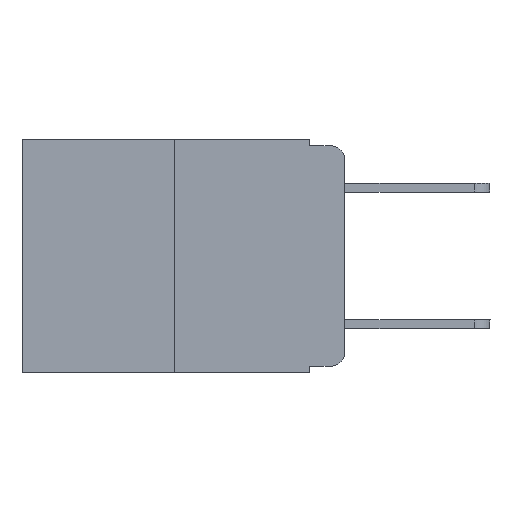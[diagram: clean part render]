
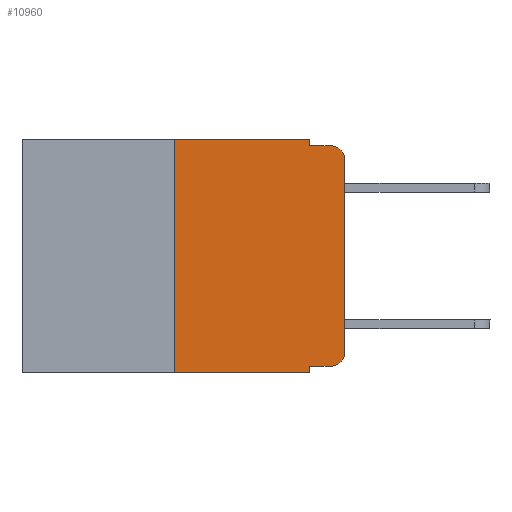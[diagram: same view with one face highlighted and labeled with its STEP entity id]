
A CAD part, left-side view. The second image highlights one B-rep face of the part: STEP entity #10960.
In plain terms, the highlighted planar face has unit normal (-1, 0, 0).
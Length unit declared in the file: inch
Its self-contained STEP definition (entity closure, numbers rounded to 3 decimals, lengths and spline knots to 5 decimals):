
#119 = LINE ( 'NONE', #8763, #12037 ) ;
#389 = VECTOR ( 'NONE', #10071, 39.37008 ) ;
#636 = CARTESIAN_POINT ( 'NONE',  ( 0., 0., -0.03 ) ) ;
#895 = DIRECTION ( 'NONE',  ( 0., 0., 1. ) ) ;
#909 = DIRECTION ( 'NONE',  ( 1., 0., 0. ) ) ;
#919 = VERTEX_POINT ( 'NONE', #2746 ) ;
#997 = CARTESIAN_POINT ( 'NONE',  ( 0., 0.473, 0. ) ) ;
#1603 = CARTESIAN_POINT ( 'NONE',  ( 0., 0.051, -0.333 ) ) ;
#1807 = LINE ( 'NONE', #5413, #7610 ) ;
#1819 = ORIENTED_EDGE ( 'NONE', *, *, #3888, .T. ) ;
#2052 = LINE ( 'NONE', #9664, #5678 ) ;
#2224 = DIRECTION ( 'NONE',  ( 0., -1., 0. ) ) ;
#2333 = CARTESIAN_POINT ( 'NONE',  ( 0., 0.051, -0.01 ) ) ;
#2435 = VERTEX_POINT ( 'NONE', #2333 ) ;
#2512 = VERTEX_POINT ( 'NONE', #636 ) ;
#2543 = DIRECTION ( 'NONE',  ( 0., 0., -1. ) ) ;
#2651 = AXIS2_PLACEMENT_3D ( 'NONE', #4947, #2930, #3047 ) ;
#2669 = CARTESIAN_POINT ( 'NONE',  ( 0., 0.02, -0.333 ) ) ;
#2746 = CARTESIAN_POINT ( 'NONE',  ( 0., 0.02, -0.01 ) ) ;
#2767 = ORIENTED_EDGE ( 'NONE', *, *, #9266, .T. ) ;
#2859 = LINE ( 'NONE', #11042, #389 ) ;
#2873 = LINE ( 'NONE', #8002, #8405 ) ;
#2891 = DIRECTION ( 'NONE',  ( 0., 0., -1. ) ) ;
#2930 = DIRECTION ( 'NONE',  ( -1., 0., 0. ) ) ;
#3047 = DIRECTION ( 'NONE',  ( 0., 0., -1. ) ) ;
#3244 = VECTOR ( 'NONE', #895, 39.37008 ) ;
#3314 = VERTEX_POINT ( 'NONE', #1603 ) ;
#3888 = EDGE_CURVE ( 'NONE', #2512, #919, #4780, .T. ) ;
#3894 = VECTOR ( 'NONE', #5170, 39.37008 ) ;
#4258 = VERTEX_POINT ( 'NONE', #10724 ) ;
#4780 = CIRCLE ( 'NONE', #5153, 0.02 ) ;
#4947 = CARTESIAN_POINT ( 'NONE',  ( 0., 0.02, -0.313 ) ) ;
#5011 = EDGE_CURVE ( 'NONE', #7599, #4258, #5187, .T. ) ;
#5047 = VERTEX_POINT ( 'NONE', #8077 ) ;
#5153 = AXIS2_PLACEMENT_3D ( 'NONE', #9343, #11237, #2891 ) ;
#5170 = DIRECTION ( 'NONE',  ( 0., 0., 1. ) ) ;
#5187 = LINE ( 'NONE', #8917, #3894 ) ;
#5374 = AXIS2_PLACEMENT_3D ( 'NONE', #997, #909, #7521 ) ;
#5413 = CARTESIAN_POINT ( 'NONE',  ( 0., 0.051, -0.01 ) ) ;
#5415 = ORIENTED_EDGE ( 'NONE', *, *, #7147, .F. ) ;
#5508 = ORIENTED_EDGE ( 'NONE', *, *, #11428, .T. ) ;
#5583 = CARTESIAN_POINT ( 'NONE',  ( 0., 0.25, -0.343 ) ) ;
#5678 = VECTOR ( 'NONE', #9786, 39.37008 ) ;
#5711 = CARTESIAN_POINT ( 'NONE',  ( 0., 0.473, 0. ) ) ;
#6020 = EDGE_CURVE ( 'NONE', #5047, #2435, #2859, .T. ) ;
#6319 = ORIENTED_EDGE ( 'NONE', *, *, #6020, .F. ) ;
#6536 = PLANE ( 'NONE',  #5374 ) ;
#6649 = DIRECTION ( 'NONE',  ( 0., -1., 0. ) ) ;
#6833 = CARTESIAN_POINT ( 'NONE',  ( 0., 0., -0.313 ) ) ;
#7147 = EDGE_CURVE ( 'NONE', #4258, #5047, #11129, .T. ) ;
#7521 = DIRECTION ( 'NONE',  ( 0., 0., -1. ) ) ;
#7543 = EDGE_CURVE ( 'NONE', #2435, #919, #1807, .T. ) ;
#7599 = VERTEX_POINT ( 'NONE', #5583 ) ;
#7610 = VECTOR ( 'NONE', #11765, 39.37008 ) ;
#7619 = EDGE_CURVE ( 'NONE', #10535, #2512, #9797, .T. ) ;
#7634 = ORIENTED_EDGE ( 'NONE', *, *, #7543, .F. ) ;
#8002 = CARTESIAN_POINT ( 'NONE',  ( 0., 0.051, 0. ) ) ;
#8077 = CARTESIAN_POINT ( 'NONE',  ( 0., 0.051, 0. ) ) ;
#8285 = ORIENTED_EDGE ( 'NONE', *, *, #8650, .T. ) ;
#8405 = VECTOR ( 'NONE', #2543, 39.37008 ) ;
#8650 = EDGE_CURVE ( 'NONE', #11829, #10535, #9035, .T. ) ;
#8763 = CARTESIAN_POINT ( 'NONE',  ( 0., 0.051, -0.333 ) ) ;
#8805 = ORIENTED_EDGE ( 'NONE', *, *, #11623, .F. ) ;
#8917 = CARTESIAN_POINT ( 'NONE',  ( 0., 0.25, 0. ) ) ;
#9035 = CIRCLE ( 'NONE', #2651, 0.02 ) ;
#9143 = VERTEX_POINT ( 'NONE', #9619 ) ;
#9266 = EDGE_CURVE ( 'NONE', #7599, #9143, #2052, .T. ) ;
#9343 = CARTESIAN_POINT ( 'NONE',  ( 0., 0.02, -0.03 ) ) ;
#9619 = CARTESIAN_POINT ( 'NONE',  ( 0., 0.051, -0.343 ) ) ;
#9664 = CARTESIAN_POINT ( 'NONE',  ( 0., 0.473, -0.343 ) ) ;
#9786 = DIRECTION ( 'NONE',  ( 0., -1., 0. ) ) ;
#9797 = LINE ( 'NONE', #11174, #3244 ) ;
#9878 = FACE_OUTER_BOUND ( 'NONE', #10505, .T. ) ;
#10071 = DIRECTION ( 'NONE',  ( 0., 0., -1. ) ) ;
#10505 = EDGE_LOOP ( 'NONE', ( #11976, #1819, #7634, #6319, #5415, #10790, #2767, #8805, #5508, #8285 ) ) ;
#10535 = VERTEX_POINT ( 'NONE', #6833 ) ;
#10724 = CARTESIAN_POINT ( 'NONE',  ( 0., 0.25, 0. ) ) ;
#10790 = ORIENTED_EDGE ( 'NONE', *, *, #5011, .F. ) ;
#10960 = ADVANCED_FACE ( 'NONE', ( #9878 ), #6536, .F. ) ;
#11042 = CARTESIAN_POINT ( 'NONE',  ( 0., 0.051, 0. ) ) ;
#11129 = LINE ( 'NONE', #5711, #11550 ) ;
#11174 = CARTESIAN_POINT ( 'NONE',  ( 0., 0., 0. ) ) ;
#11237 = DIRECTION ( 'NONE',  ( -1., 0., 0. ) ) ;
#11428 = EDGE_CURVE ( 'NONE', #3314, #11829, #119, .T. ) ;
#11550 = VECTOR ( 'NONE', #6649, 39.37008 ) ;
#11623 = EDGE_CURVE ( 'NONE', #3314, #9143, #2873, .T. ) ;
#11765 = DIRECTION ( 'NONE',  ( 0., -1., 0. ) ) ;
#11829 = VERTEX_POINT ( 'NONE', #2669 ) ;
#11976 = ORIENTED_EDGE ( 'NONE', *, *, #7619, .T. ) ;
#12037 = VECTOR ( 'NONE', #2224, 39.37008 ) ;
